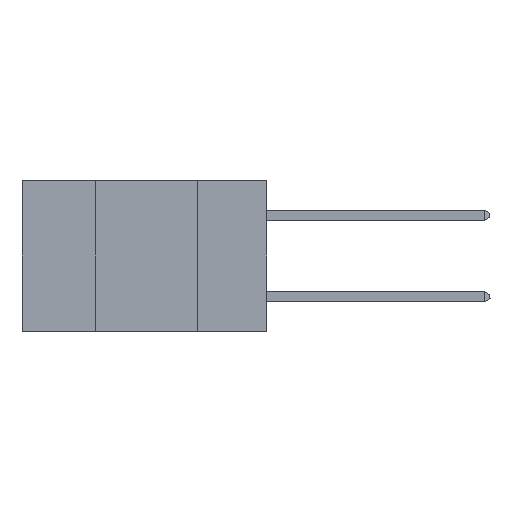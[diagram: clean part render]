
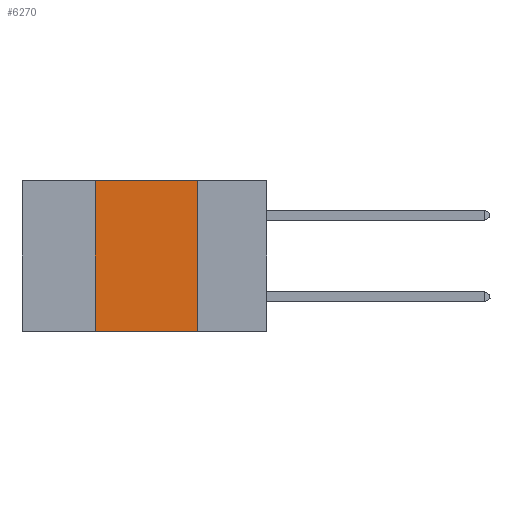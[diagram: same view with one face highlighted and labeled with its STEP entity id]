
A CAD part, left-side view. The second image highlights one B-rep face of the part: STEP entity #6270.
In plain terms, the highlighted planar face has unit normal (-1, 0, 0).
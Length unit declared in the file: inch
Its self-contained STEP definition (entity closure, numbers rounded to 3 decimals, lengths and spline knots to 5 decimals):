
#467 = CARTESIAN_POINT ( 'NONE',  ( 0., 0.17, 0. ) ) ;
#1019 = EDGE_LOOP ( 'NONE', ( #12719, #11288, #9547, #7657 ) ) ;
#1607 = DIRECTION ( 'NONE',  ( 0., 0., -1. ) ) ;
#1911 = VERTEX_POINT ( 'NONE', #2762 ) ;
#1925 = DIRECTION ( 'NONE',  ( 1., 0., 0. ) ) ;
#2487 = LINE ( 'NONE', #3140, #7368 ) ;
#2762 = CARTESIAN_POINT ( 'NONE',  ( 0., 0.42, -0.37 ) ) ;
#2803 = CARTESIAN_POINT ( 'NONE',  ( 0., 0.6, -0.37 ) ) ;
#2991 = CARTESIAN_POINT ( 'NONE',  ( 0., 0.6, 0. ) ) ;
#3140 = CARTESIAN_POINT ( 'NONE',  ( 0., 0.42, 0. ) ) ;
#3880 = DIRECTION ( 'NONE',  ( 0., -1., 0. ) ) ;
#4216 = DIRECTION ( 'NONE',  ( 0., 0., 1. ) ) ;
#5011 = AXIS2_PLACEMENT_3D ( 'NONE', #2991, #1925, #9195 ) ;
#5118 = PLANE ( 'NONE',  #5011 ) ;
#5337 = CARTESIAN_POINT ( 'NONE',  ( 0., 0.6, 0. ) ) ;
#5509 = FACE_OUTER_BOUND ( 'NONE', #1019, .T. ) ;
#5526 = CARTESIAN_POINT ( 'NONE',  ( 0., 0.42, 0. ) ) ;
#6127 = EDGE_CURVE ( 'NONE', #1911, #9053, #10084, .T. ) ;
#6270 = ADVANCED_FACE ( 'NONE', ( #5509 ), #5118, .F. ) ;
#7368 = VECTOR ( 'NONE', #4216, 39.37008 ) ;
#7657 = ORIENTED_EDGE ( 'NONE', *, *, #6127, .T. ) ;
#7712 = CARTESIAN_POINT ( 'NONE',  ( 0., 0.17, -0.37 ) ) ;
#8121 = LINE ( 'NONE', #467, #13497 ) ;
#8406 = DIRECTION ( 'NONE',  ( 0., -1., 0. ) ) ;
#8854 = EDGE_CURVE ( 'NONE', #1911, #10930, #2487, .T. ) ;
#9053 = VERTEX_POINT ( 'NONE', #7712 ) ;
#9195 = DIRECTION ( 'NONE',  ( 0., 0., -1. ) ) ;
#9452 = EDGE_CURVE ( 'NONE', #10930, #9659, #12099, .T. ) ;
#9547 = ORIENTED_EDGE ( 'NONE', *, *, #8854, .F. ) ;
#9659 = VERTEX_POINT ( 'NONE', #12790 ) ;
#9785 = VECTOR ( 'NONE', #3880, 39.37008 ) ;
#10084 = LINE ( 'NONE', #2803, #9785 ) ;
#10930 = VERTEX_POINT ( 'NONE', #5526 ) ;
#11288 = ORIENTED_EDGE ( 'NONE', *, *, #9452, .F. ) ;
#12099 = LINE ( 'NONE', #5337, #13203 ) ;
#12719 = ORIENTED_EDGE ( 'NONE', *, *, #12933, .F. ) ;
#12790 = CARTESIAN_POINT ( 'NONE',  ( 0., 0.17, 0. ) ) ;
#12933 = EDGE_CURVE ( 'NONE', #9659, #9053, #8121, .T. ) ;
#13203 = VECTOR ( 'NONE', #8406, 39.37008 ) ;
#13497 = VECTOR ( 'NONE', #1607, 39.37008 ) ;
